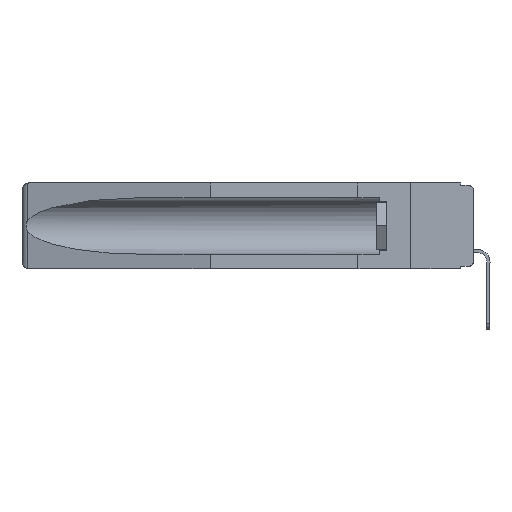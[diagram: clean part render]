
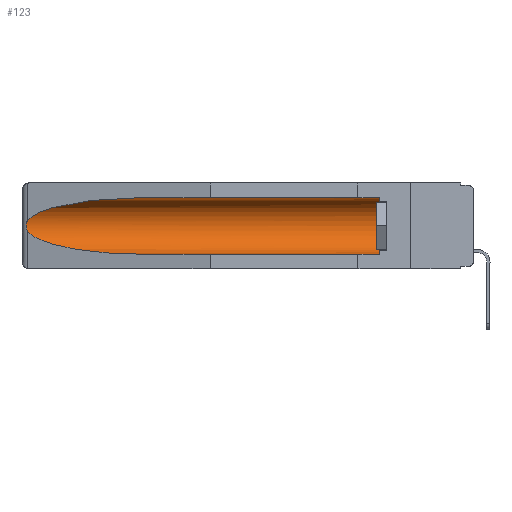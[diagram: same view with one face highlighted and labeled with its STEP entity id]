
A CAD part, left-side view. The second image highlights one B-rep face of the part: STEP entity #123.
In plain terms, the highlighted cylindrical face has radius 2.857 mm (diameter 5.715 mm), a partial arc.
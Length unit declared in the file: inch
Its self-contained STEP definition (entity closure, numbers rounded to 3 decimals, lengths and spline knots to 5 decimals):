
#123 = ADVANCED_FACE ( 'NONE', ( #145 ), #6401, .F. ) ;
#145 = FACE_OUTER_BOUND ( 'NONE', #12274, .T. ) ;
#268 = VERTEX_POINT ( 'NONE', #7528 ) ;
#795 = CARTESIAN_POINT ( 'NONE',  ( 0.26537, 1.52718, -0.14972 ) ) ;
#1005 = LINE ( 'NONE', #16545, #10270 ) ;
#1497 = CARTESIAN_POINT ( 'NONE',  ( 0.155, 1.07973, -0.284 ) ) ;
#1703 = EDGE_CURVE ( 'NONE', #15122, #268, #15665, .T. ) ;
#3032 = CARTESIAN_POINT ( 'NONE',  ( 0.26537, 1.52718, -0.19328 ) ) ;
#3615 = CARTESIAN_POINT ( 'NONE',  ( 0.155, -0.30754, -0.284 ) ) ;
#3620 = CARTESIAN_POINT ( 'NONE',  ( 0.2675, 1.53308, -0.16763 ) ) ;
#3671 = CARTESIAN_POINT ( 'NONE',  ( 0.155, 0.126, -0.1715 ) ) ;
#3723 = CARTESIAN_POINT ( 'NONE',  ( 0.26655, 1.53094, -0.18657 ) ) ;
#4246 = CARTESIAN_POINT ( 'NONE',  ( 0.155, 1.07973, -0.059 ) ) ;
#4389 = VERTEX_POINT ( 'NONE', #8934 ) ;
#4640 = EDGE_CURVE ( 'NONE', #4389, #9709, #16384, .T. ) ;
#4668 = CARTESIAN_POINT ( 'NONE',  ( 0.25451, 1.48313, -0.24835 ) ) ;
#5153 = CARTESIAN_POINT ( 'NONE',  ( 0.2673, 1.5327, -0.16383 ) ) ;
#5876 = EDGE_CURVE ( 'NONE', #11849, #15122, #18033, .T. ) ;
#5881 =( BOUNDED_CURVE ( )  B_SPLINE_CURVE ( 3, ( #8287, #19202, #14612, #795 ),
 .UNSPECIFIED., .F., .F. ) 
 B_SPLINE_CURVE_WITH_KNOTS ( ( 4, 4 ),
 ( 4.71239, 6.08839 ),
 .UNSPECIFIED. ) 
 CURVE ( )  GEOMETRIC_REPRESENTATION_ITEM ( )  RATIONAL_B_SPLINE_CURVE ( ( 1., 0.848, 0.848, 1. ) ) 
 REPRESENTATION_ITEM ( '' )  );
#6311 = ORIENTED_EDGE ( 'NONE', *, *, #5876, .T. ) ;
#6401 = CYLINDRICAL_SURFACE ( 'NONE', #13410, 0.1125 ) ;
#7064 = DIRECTION ( 'NONE',  ( 0., 0., 1. ) ) ;
#7234 = ORIENTED_EDGE ( 'NONE', *, *, #16460, .F. ) ;
#7528 = CARTESIAN_POINT ( 'NONE',  ( 0.155, 1.07973, -0.284 ) ) ;
#8042 = CARTESIAN_POINT ( 'NONE',  ( 0.2675, 1.53308, -0.17534 ) ) ;
#8249 = CARTESIAN_POINT ( 'NONE',  ( 0.26597, 1.5296, -0.19026 ) ) ;
#8287 = CARTESIAN_POINT ( 'NONE',  ( 0.155, 1.07973, -0.059 ) ) ;
#8439 = DIRECTION ( 'NONE',  ( 0., 1., 0. ) ) ;
#8934 = CARTESIAN_POINT ( 'NONE',  ( 0.155, 0.126, -0.284 ) ) ;
#9477 = CARTESIAN_POINT ( 'NONE',  ( 0.21114, 1.30732, -0.284 ) ) ;
#9709 = VERTEX_POINT ( 'NONE', #13605 ) ;
#10270 = VECTOR ( 'NONE', #16762, 39.37008 ) ;
#10611 = VERTEX_POINT ( 'NONE', #4246 ) ;
#11116 = ORIENTED_EDGE ( 'NONE', *, *, #14313, .T. ) ;
#11289 = CARTESIAN_POINT ( 'NONE',  ( 0.26537, 1.52718, -0.19328 ) ) ;
#11391 = CARTESIAN_POINT ( 'NONE',  ( 0.2673, 1.53269, -0.17917 ) ) ;
#11446 = ORIENTED_EDGE ( 'NONE', *, *, #4640, .T. ) ;
#11595 = LINE ( 'NONE', #3615, #18057 ) ;
#11600 = CARTESIAN_POINT ( 'NONE',  ( 0.26597, 1.52961, -0.15275 ) ) ;
#11849 = VERTEX_POINT ( 'NONE', #12022 ) ;
#12022 = CARTESIAN_POINT ( 'NONE',  ( 0.26537, 1.52718, -0.14972 ) ) ;
#12274 = EDGE_LOOP ( 'NONE', ( #11116, #6311, #16425, #7234, #11446, #14993 ) ) ;
#12627 = CARTESIAN_POINT ( 'NONE',  ( 0.155, -0.30754, -0.1715 ) ) ;
#13028 = CARTESIAN_POINT ( 'NONE',  ( 0.26654, 1.53092, -0.15636 ) ) ;
#13410 = AXIS2_PLACEMENT_3D ( 'NONE', #12627, #18863, #17326 ) ;
#13605 = CARTESIAN_POINT ( 'NONE',  ( 0.155, 0.126, -0.059 ) ) ;
#14313 = EDGE_CURVE ( 'NONE', #10611, #11849, #5881, .T. ) ;
#14612 = CARTESIAN_POINT ( 'NONE',  ( 0.25451, 1.48313, -0.09465 ) ) ;
#14993 = ORIENTED_EDGE ( 'NONE', *, *, #17587, .T. ) ;
#15122 = VERTEX_POINT ( 'NONE', #16061 ) ;
#15665 =( BOUNDED_CURVE ( )  B_SPLINE_CURVE ( 3, ( #3032, #4668, #9477, #1497 ),
 .UNSPECIFIED., .F., .F. ) 
 B_SPLINE_CURVE_WITH_KNOTS ( ( 4, 4 ),
 ( 0.1948, 1.5708 ),
 .UNSPECIFIED. ) 
 CURVE ( )  GEOMETRIC_REPRESENTATION_ITEM ( )  RATIONAL_B_SPLINE_CURVE ( ( 1., 0.848, 0.848, 1. ) ) 
 REPRESENTATION_ITEM ( '' )  );
#16061 = CARTESIAN_POINT ( 'NONE',  ( 0.26537, 1.52718, -0.19328 ) ) ;
#16384 = CIRCLE ( 'NONE', #19367, 0.1125 ) ;
#16425 = ORIENTED_EDGE ( 'NONE', *, *, #1703, .T. ) ;
#16460 = EDGE_CURVE ( 'NONE', #4389, #268, #11595, .T. ) ;
#16545 = CARTESIAN_POINT ( 'NONE',  ( 0.155, -0.30754, -0.059 ) ) ;
#16762 = DIRECTION ( 'NONE',  ( 0., 1., 0. ) ) ;
#17326 = DIRECTION ( 'NONE',  ( 0., 0., 1. ) ) ;
#17587 = EDGE_CURVE ( 'NONE', #9709, #10611, #1005, .T. ) ;
#18033 = B_SPLINE_CURVE_WITH_KNOTS ( 'NONE', 3,
 ( #19163, #11600, #13028, #5153, #3620, #8042, #11391, #3723, #8249, #11289 ),
 .UNSPECIFIED., .F., .F.,
 ( 4, 2, 2, 2, 4 ),
 ( 0., 0.00029, 0.00058, 0.00087, 0.00117 ),
 .UNSPECIFIED. ) ;
#18057 = VECTOR ( 'NONE', #8439, 39.37008 ) ;
#18863 = DIRECTION ( 'NONE',  ( 0., 1., 0. ) ) ;
#19163 = CARTESIAN_POINT ( 'NONE',  ( 0.26537, 1.52718, -0.14972 ) ) ;
#19202 = CARTESIAN_POINT ( 'NONE',  ( 0.21114, 1.30732, -0.059 ) ) ;
#19211 = DIRECTION ( 'NONE',  ( 0., -1., 0. ) ) ;
#19367 = AXIS2_PLACEMENT_3D ( 'NONE', #3671, #19211, #7064 ) ;
